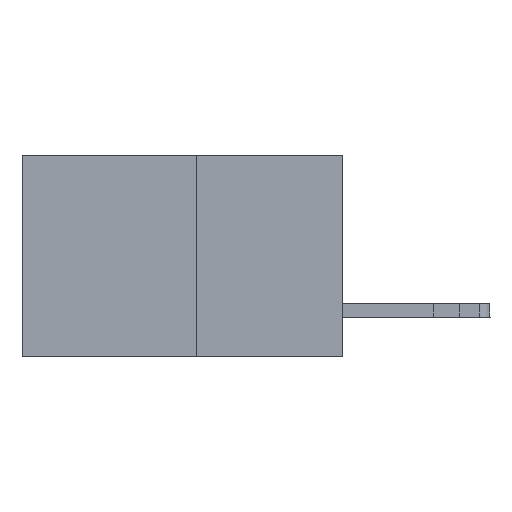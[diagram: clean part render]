
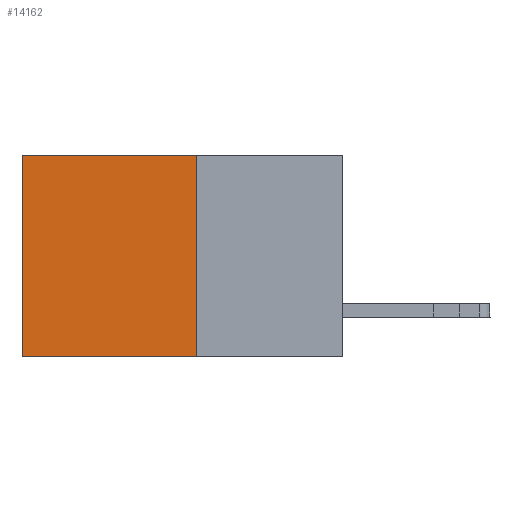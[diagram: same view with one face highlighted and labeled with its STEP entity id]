
A CAD part, left-side view. The second image highlights one B-rep face of the part: STEP entity #14162.
In plain terms, the highlighted planar face has unit normal (-1, 0, 0).
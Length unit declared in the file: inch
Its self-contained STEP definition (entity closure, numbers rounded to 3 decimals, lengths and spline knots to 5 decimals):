
#171 = AXIS2_PLACEMENT_3D ( 'NONE', #2478, #182, #16780 ) ;
#182 = DIRECTION ( 'NONE',  ( 1., 0., 0. ) ) ;
#570 = VECTOR ( 'NONE', #5909, 39.37008 ) ;
#729 = CARTESIAN_POINT ( 'NONE',  ( 0.277, 0.27, -0.37 ) ) ;
#1065 = CARTESIAN_POINT ( 'NONE',  ( 0.277, 0.27, -0.37 ) ) ;
#1839 = LINE ( 'NONE', #5577, #570 ) ;
#1982 = VERTEX_POINT ( 'NONE', #7938 ) ;
#2478 = CARTESIAN_POINT ( 'NONE',  ( 0.277, 0.27, -0.37 ) ) ;
#3745 = CARTESIAN_POINT ( 'NONE',  ( 0.277, 0.59, -0.37 ) ) ;
#4097 = FACE_OUTER_BOUND ( 'NONE', #5930, .T. ) ;
#4247 = VECTOR ( 'NONE', #5566, 39.37008 ) ;
#4684 = CARTESIAN_POINT ( 'NONE',  ( 0.277, 0.59, 0. ) ) ;
#5270 = CARTESIAN_POINT ( 'NONE',  ( 0.277, 0.59, -0.37 ) ) ;
#5566 = DIRECTION ( 'NONE',  ( 0., 1., 0. ) ) ;
#5577 = CARTESIAN_POINT ( 'NONE',  ( 0.277, 0.27, -0.37 ) ) ;
#5724 = EDGE_CURVE ( 'NONE', #15460, #8198, #7192, .T. ) ;
#5909 = DIRECTION ( 'NONE',  ( 0., 0., -1. ) ) ;
#5930 = EDGE_LOOP ( 'NONE', ( #7920, #10402, #8188, #7569 ) ) ;
#6928 = CARTESIAN_POINT ( 'NONE',  ( 0.277, 0.27, 0. ) ) ;
#7192 = LINE ( 'NONE', #729, #8532 ) ;
#7569 = ORIENTED_EDGE ( 'NONE', *, *, #15196, .T. ) ;
#7920 = ORIENTED_EDGE ( 'NONE', *, *, #14244, .T. ) ;
#7938 = CARTESIAN_POINT ( 'NONE',  ( 0.277, 0.27, 0. ) ) ;
#8188 = ORIENTED_EDGE ( 'NONE', *, *, #10231, .F. ) ;
#8198 = VERTEX_POINT ( 'NONE', #3745 ) ;
#8532 = VECTOR ( 'NONE', #9195, 39.37008 ) ;
#9034 = DIRECTION ( 'NONE',  ( 0., 0., -1. ) ) ;
#9195 = DIRECTION ( 'NONE',  ( 0., 1., 0. ) ) ;
#9482 = VERTEX_POINT ( 'NONE', #4684 ) ;
#10231 = EDGE_CURVE ( 'NONE', #1982, #15460, #1839, .T. ) ;
#10402 = ORIENTED_EDGE ( 'NONE', *, *, #5724, .F. ) ;
#11863 = VECTOR ( 'NONE', #9034, 39.37008 ) ;
#12130 = LINE ( 'NONE', #6928, #4247 ) ;
#12786 = PLANE ( 'NONE',  #171 ) ;
#12863 = LINE ( 'NONE', #5270, #11863 ) ;
#14162 = ADVANCED_FACE ( 'NONE', ( #4097 ), #12786, .F. ) ;
#14244 = EDGE_CURVE ( 'NONE', #9482, #8198, #12863, .T. ) ;
#15196 = EDGE_CURVE ( 'NONE', #1982, #9482, #12130, .T. ) ;
#15460 = VERTEX_POINT ( 'NONE', #1065 ) ;
#16780 = DIRECTION ( 'NONE',  ( 0., 0., -1. ) ) ;
